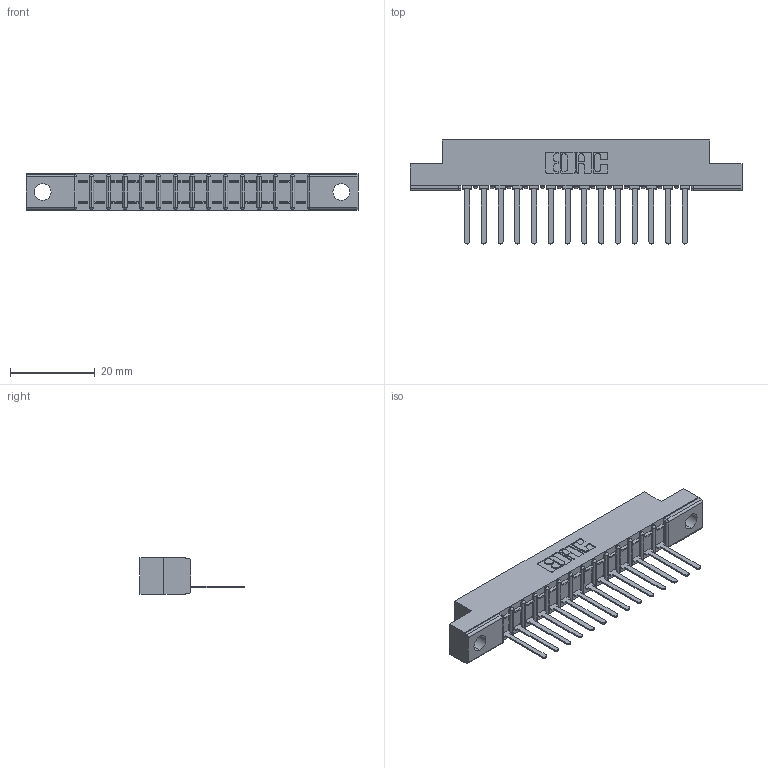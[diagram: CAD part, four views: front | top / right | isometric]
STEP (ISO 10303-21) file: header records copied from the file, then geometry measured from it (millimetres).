
FILE_DESCRIPTION (( 'STEP AP203' ), '1' );
FILE_NAME ('307-014-441-104.STEP', '2020-09-25T15:49:03', ( '' ), ( '' ), 'SwSTEP 2.0', 'SolidWorks 2020', '' );
FILE_SCHEMA (( 'CONFIG_CONTROL_DESIGN' ));
Length unit declared in the file: inch
Products named in the file (3): 307 Part_.156 Dia Mounting Holes; 307-014-441-104; 307-290-002_541
Assembly tree (15 placements, depth 2):
  307-014-441-104
    307 Part_.156 Dia Mounting Holes
    307-290-002_541  x14
Bounding box: 78.49 x 24.59 x 8.71 mm (x, y, z)
Volume: 5110.9 mm3; surface area: 8980.3 mm2
Topology: 15 solids, 15 shells, 1183 faces, 3607 edges, 2362 vertices
Faces by surface type: plane 714, cylinder 439, sphere 30
Entity records: 16590 total; most frequent: CARTESIAN_POINT 2798, ORIENTED_EDGE 2786, DIRECTION 2723, EDGE_CURVE 1393, VECTOR 1061, LINE 1061, VERTEX_POINT 906, AXIS2_PLACEMENT_3D 831
